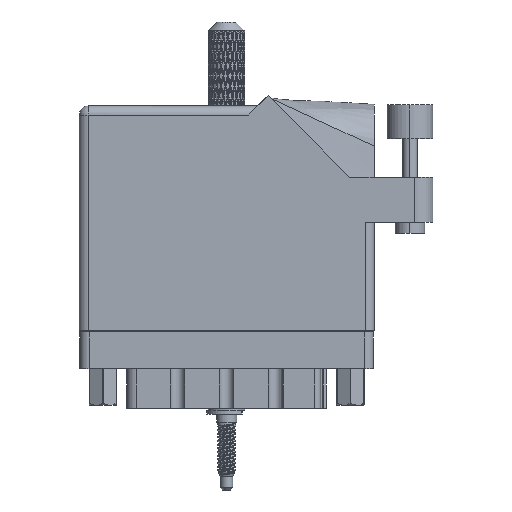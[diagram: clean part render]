
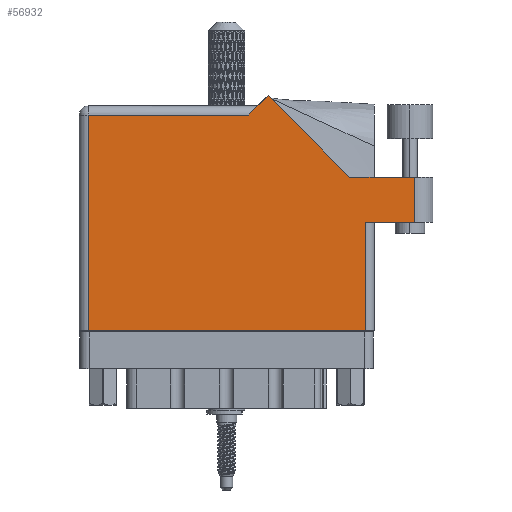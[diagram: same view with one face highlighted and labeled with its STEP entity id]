
A CAD part, front view. The second image highlights one B-rep face of the part: STEP entity #56932.
In plain terms, the highlighted face is planar.
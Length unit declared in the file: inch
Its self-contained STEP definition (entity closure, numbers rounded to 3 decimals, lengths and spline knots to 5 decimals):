
#991 = DIRECTION ( 'NONE',  ( -1., 0., 0. ) ) ;
#1567 = CARTESIAN_POINT ( 'NONE',  ( 0., 1.468, 0. ) ) ;
#2348 = CARTESIAN_POINT ( 'NONE',  ( 1.84442, 1.044, 0. ) ) ;
#4766 = LINE ( 'NONE', #49849, #65155 ) ;
#5907 = DIRECTION ( 'NONE',  ( 0., -1., 0. ) ) ;
#6186 = CARTESIAN_POINT ( 'NONE',  ( 1.948, 0.737, 0. ) ) ;
#8356 = VECTOR ( 'NONE', #61289, 39.37008 ) ;
#10681 = ORIENTED_EDGE ( 'NONE', *, *, #62663, .T. ) ;
#11382 = VECTOR ( 'NONE', #71011, 39.37008 ) ;
#11656 = ORIENTED_EDGE ( 'NONE', *, *, #53532, .T. ) ;
#15422 = DIRECTION ( 'NONE',  ( 1., 0., 0. ) ) ;
#20047 = EDGE_CURVE ( 'NONE', #106650, #50286, #86477, .T. ) ;
#22128 = ORIENTED_EDGE ( 'NONE', *, *, #85110, .T. ) ;
#22191 = ORIENTED_EDGE ( 'NONE', *, *, #101808, .T. ) ;
#23782 = ORIENTED_EDGE ( 'NONE', *, *, #20047, .T. ) ;
#28895 = VERTEX_POINT ( 'NONE', #32259 ) ;
#29325 = DIRECTION ( 'NONE',  ( -0.707, 0.707, 0. ) ) ;
#32259 = CARTESIAN_POINT ( 'NONE',  ( 1.155, 1.468, 0. ) ) ;
#34916 = DIRECTION ( 'NONE',  ( 0., 0., -1. ) ) ;
#35475 = VERTEX_POINT ( 'NONE', #64652 ) ;
#35608 = LINE ( 'NONE', #1567, #60695 ) ;
#39402 = LINE ( 'NONE', #48164, #104876 ) ;
#42509 = EDGE_CURVE ( 'NONE', #35475, #106810, #4766, .T. ) ;
#42586 = CARTESIAN_POINT ( 'NONE',  ( 2.41, 1.044, 0. ) ) ;
#43110 = CARTESIAN_POINT ( 'NONE',  ( 0., 1.53, 0. ) ) ;
#43535 = LINE ( 'NONE', #70435, #11382 ) ;
#44019 = DIRECTION ( 'NONE',  ( 1., 0., 0. ) ) ;
#45121 = VERTEX_POINT ( 'NONE', #47400 ) ;
#46101 = CARTESIAN_POINT ( 'NONE',  ( 1.84442, 1.044, 0. ) ) ;
#47400 = CARTESIAN_POINT ( 'NONE',  ( 2.285, 0.737, 0. ) ) ;
#48164 = CARTESIAN_POINT ( 'NONE',  ( 2.285, 1.044, 0. ) ) ;
#49837 = VERTEX_POINT ( 'NONE', #86679 ) ;
#49849 = CARTESIAN_POINT ( 'NONE',  ( 0.062, 0., 0. ) ) ;
#50286 = VERTEX_POINT ( 'NONE', #46101 ) ;
#51352 = ORIENTED_EDGE ( 'NONE', *, *, #78537, .T. ) ;
#51536 = EDGE_CURVE ( 'NONE', #106810, #49837, #85095, .T. ) ;
#51737 = EDGE_CURVE ( 'NONE', #59023, #28895, #43535, .T. ) ;
#53532 = EDGE_CURVE ( 'NONE', #45121, #106650, #39402, .T. ) ;
#53604 = EDGE_LOOP ( 'NONE', ( #22128, #11656, #23782, #22191, #75634, #10681, #95390, #110510, #51352 ) ) ;
#54601 = CARTESIAN_POINT ( 'NONE',  ( 1.948, 0.737, 0. ) ) ;
#56046 = CARTESIAN_POINT ( 'NONE',  ( 0.062, 0., 0. ) ) ;
#56493 = VECTOR ( 'NONE', #44019, 39.37008 ) ;
#56932 = ADVANCED_FACE ( 'NONE', ( #70595 ), #61233, .F. ) ;
#59023 = VERTEX_POINT ( 'NONE', #76835 ) ;
#59849 = VECTOR ( 'NONE', #15422, 39.37008 ) ;
#60695 = VECTOR ( 'NONE', #991, 39.37008 ) ;
#61233 = PLANE ( 'NONE',  #92121 ) ;
#61289 = DIRECTION ( 'NONE',  ( -1., 0., 0. ) ) ;
#61572 = LINE ( 'NONE', #69200, #56493 ) ;
#62663 = EDGE_CURVE ( 'NONE', #28895, #35475, #35608, .T. ) ;
#64652 = CARTESIAN_POINT ( 'NONE',  ( 0.062, 1.468, 0. ) ) ;
#65155 = VECTOR ( 'NONE', #5907, 39.37008 ) ;
#65161 = DIRECTION ( 'NONE',  ( 0., 1., 0. ) ) ;
#69200 = CARTESIAN_POINT ( 'NONE',  ( 2.01, 0.737, 0. ) ) ;
#70435 = CARTESIAN_POINT ( 'NONE',  ( 1.217, 1.53, 0. ) ) ;
#70595 = FACE_OUTER_BOUND ( 'NONE', #53604, .T. ) ;
#71011 = DIRECTION ( 'NONE',  ( -0.707, -0.707, 0. ) ) ;
#71038 = VECTOR ( 'NONE', #100800, 39.37008 ) ;
#75634 = ORIENTED_EDGE ( 'NONE', *, *, #51737, .T. ) ;
#76835 = CARTESIAN_POINT ( 'NONE',  ( 1.28771, 1.60071, 0. ) ) ;
#78537 = EDGE_CURVE ( 'NONE', #49837, #96867, #92626, .T. ) ;
#85095 = LINE ( 'NONE', #113738, #59849 ) ;
#85110 = EDGE_CURVE ( 'NONE', #96867, #45121, #61572, .T. ) ;
#86477 = LINE ( 'NONE', #42586, #8356 ) ;
#86679 = CARTESIAN_POINT ( 'NONE',  ( 1.948, 0., 0. ) ) ;
#86994 = DIRECTION ( 'NONE',  ( -1., 0., 0. ) ) ;
#92121 = AXIS2_PLACEMENT_3D ( 'NONE', #43110, #34916, #86994 ) ;
#92626 = LINE ( 'NONE', #54601, #71038 ) ;
#95390 = ORIENTED_EDGE ( 'NONE', *, *, #42509, .T. ) ;
#96867 = VERTEX_POINT ( 'NONE', #6186 ) ;
#100800 = DIRECTION ( 'NONE',  ( 0., 1., 0. ) ) ;
#101808 = EDGE_CURVE ( 'NONE', #50286, #59023, #110053, .T. ) ;
#104876 = VECTOR ( 'NONE', #65161, 39.37008 ) ;
#106431 = VECTOR ( 'NONE', #29325, 39.37008 ) ;
#106650 = VERTEX_POINT ( 'NONE', #108736 ) ;
#106810 = VERTEX_POINT ( 'NONE', #56046 ) ;
#108736 = CARTESIAN_POINT ( 'NONE',  ( 2.285, 1.044, 0. ) ) ;
#110053 = LINE ( 'NONE', #2348, #106431 ) ;
#110510 = ORIENTED_EDGE ( 'NONE', *, *, #51536, .T. ) ;
#113738 = CARTESIAN_POINT ( 'NONE',  ( 0., 0., 0. ) ) ;
